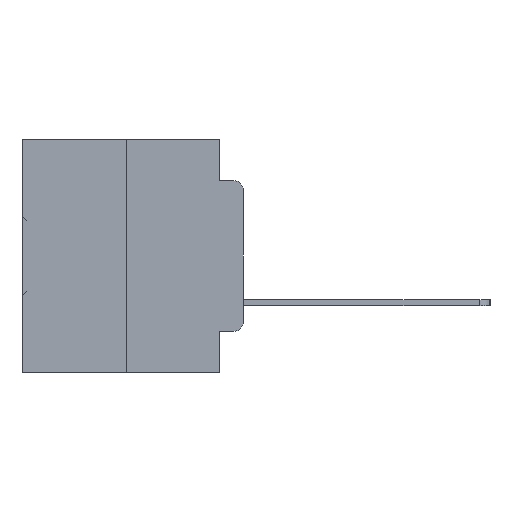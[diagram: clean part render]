
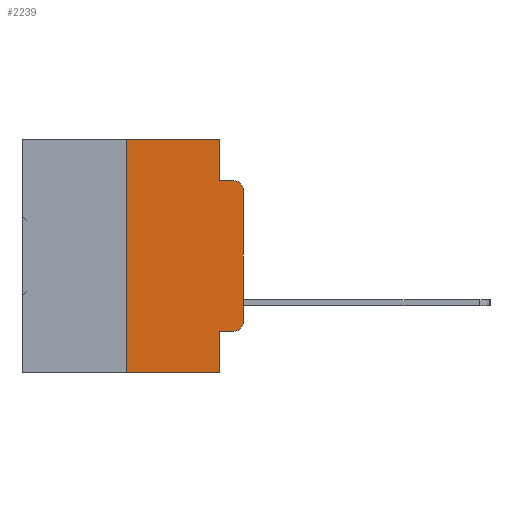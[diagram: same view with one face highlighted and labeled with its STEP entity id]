
A CAD part, left-side view. The second image highlights one B-rep face of the part: STEP entity #2239.
In plain terms, the highlighted planar face has unit normal (-1, 0, 0).
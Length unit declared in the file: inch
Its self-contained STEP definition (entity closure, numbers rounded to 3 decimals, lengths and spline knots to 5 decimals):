
#997 = CARTESIAN_POINT ( 'NONE',  ( 0., 0.051, 0. ) ) ;
#1049 = VECTOR ( 'NONE', #16141, 39.37008 ) ;
#1547 = CIRCLE ( 'NONE', #30281, 0.02 ) ;
#1980 = EDGE_CURVE ( 'NONE', #6962, #26401, #17371, .T. ) ;
#2239 = ADVANCED_FACE ( 'NONE', ( #8444 ), #26455, .F. ) ;
#2429 = CARTESIAN_POINT ( 'NONE',  ( 0., 0.02, -0.1085 ) ) ;
#3225 = DIRECTION ( 'NONE',  ( -1., 0., 0. ) ) ;
#4237 = ORIENTED_EDGE ( 'NONE', *, *, #25578, .T. ) ;
#5030 = VERTEX_POINT ( 'NONE', #24433 ) ;
#5188 = VERTEX_POINT ( 'NONE', #13718 ) ;
#5341 = DIRECTION ( 'NONE',  ( 0., 0., -1. ) ) ;
#5739 = LINE ( 'NONE', #11462, #27465 ) ;
#6173 = LINE ( 'NONE', #27408, #26995 ) ;
#6200 = CARTESIAN_POINT ( 'NONE',  ( 0., 0.25, -0.5 ) ) ;
#6962 = VERTEX_POINT ( 'NONE', #7431 ) ;
#7214 = AXIS2_PLACEMENT_3D ( 'NONE', #20327, #3225, #23152 ) ;
#7288 = EDGE_CURVE ( 'NONE', #20079, #12696, #6173, .T. ) ;
#7431 = CARTESIAN_POINT ( 'NONE',  ( 0., 0.051, -0.4115 ) ) ;
#8252 = ORIENTED_EDGE ( 'NONE', *, *, #18766, .F. ) ;
#8444 = FACE_OUTER_BOUND ( 'NONE', #18345, .T. ) ;
#9199 = VERTEX_POINT ( 'NONE', #16637 ) ;
#9773 = EDGE_CURVE ( 'NONE', #5188, #16081, #17669, .T. ) ;
#9818 = VECTOR ( 'NONE', #31308, 39.37008 ) ;
#11427 = ORIENTED_EDGE ( 'NONE', *, *, #23356, .T. ) ;
#11462 = CARTESIAN_POINT ( 'NONE',  ( 0., 0., 0. ) ) ;
#12016 = LINE ( 'NONE', #997, #26105 ) ;
#12602 = CARTESIAN_POINT ( 'NONE',  ( 0., 0., -0.1085 ) ) ;
#12696 = VERTEX_POINT ( 'NONE', #33293 ) ;
#13718 = CARTESIAN_POINT ( 'NONE',  ( 0., 0.25, 0. ) ) ;
#14218 = LINE ( 'NONE', #17754, #20815 ) ;
#14300 = CIRCLE ( 'NONE', #7214, 0.02 ) ;
#16081 = VERTEX_POINT ( 'NONE', #24579 ) ;
#16141 = DIRECTION ( 'NONE',  ( 0., -1., 0. ) ) ;
#16235 = DIRECTION ( 'NONE',  ( 0., -1., 0. ) ) ;
#16310 = ORIENTED_EDGE ( 'NONE', *, *, #16898, .F. ) ;
#16349 = ORIENTED_EDGE ( 'NONE', *, *, #26290, .F. ) ;
#16637 = CARTESIAN_POINT ( 'NONE',  ( 0., 0.051, -0.5 ) ) ;
#16790 = VECTOR ( 'NONE', #16235, 39.37008 ) ;
#16898 = EDGE_CURVE ( 'NONE', #16081, #20079, #33378, .T. ) ;
#17371 = LINE ( 'NONE', #33043, #9818 ) ;
#17664 = CARTESIAN_POINT ( 'NONE',  ( 0., 0.051, 0. ) ) ;
#17669 = LINE ( 'NONE', #24572, #16790 ) ;
#17754 = CARTESIAN_POINT ( 'NONE',  ( 0., 0.25, 0. ) ) ;
#18345 = EDGE_LOOP ( 'NONE', ( #11427, #32995, #31238, #16310, #24193, #8252, #22427, #16349, #35174, #4237 ) ) ;
#18766 = EDGE_CURVE ( 'NONE', #35471, #5188, #14218, .T. ) ;
#19142 = EDGE_CURVE ( 'NONE', #32050, #12696, #1547, .T. ) ;
#19979 = DIRECTION ( 'NONE',  ( 0., 0., 1. ) ) ;
#20079 = VERTEX_POINT ( 'NONE', #20961 ) ;
#20327 = CARTESIAN_POINT ( 'NONE',  ( 0., 0.02, -0.3915 ) ) ;
#20815 = VECTOR ( 'NONE', #34530, 39.37008 ) ;
#20961 = CARTESIAN_POINT ( 'NONE',  ( 0., 0.051, -0.0885 ) ) ;
#22370 = DIRECTION ( 'NONE',  ( -1., 0., 0. ) ) ;
#22427 = ORIENTED_EDGE ( 'NONE', *, *, #28146, .T. ) ;
#23152 = DIRECTION ( 'NONE',  ( 0., 0., -1. ) ) ;
#23298 = DIRECTION ( 'NONE',  ( 0., 0., -1. ) ) ;
#23356 = EDGE_CURVE ( 'NONE', #5030, #32050, #5739, .T. ) ;
#23667 = AXIS2_PLACEMENT_3D ( 'NONE', #31352, #30116, #32804 ) ;
#23840 = DIRECTION ( 'NONE',  ( 0., 0., -1. ) ) ;
#24193 = ORIENTED_EDGE ( 'NONE', *, *, #9773, .F. ) ;
#24433 = CARTESIAN_POINT ( 'NONE',  ( 0., 0., -0.3915 ) ) ;
#24572 = CARTESIAN_POINT ( 'NONE',  ( 0., 0.473, 0. ) ) ;
#24579 = CARTESIAN_POINT ( 'NONE',  ( 0., 0.051, 0. ) ) ;
#25578 = EDGE_CURVE ( 'NONE', #26401, #5030, #14300, .T. ) ;
#26105 = VECTOR ( 'NONE', #23840, 39.37008 ) ;
#26290 = EDGE_CURVE ( 'NONE', #6962, #9199, #12016, .T. ) ;
#26401 = VERTEX_POINT ( 'NONE', #27132 ) ;
#26455 = PLANE ( 'NONE',  #23667 ) ;
#26995 = VECTOR ( 'NONE', #27290, 39.37008 ) ;
#27132 = CARTESIAN_POINT ( 'NONE',  ( 0., 0.02, -0.4115 ) ) ;
#27290 = DIRECTION ( 'NONE',  ( 0., -1., 0. ) ) ;
#27408 = CARTESIAN_POINT ( 'NONE',  ( 0., 0.051, -0.0885 ) ) ;
#27465 = VECTOR ( 'NONE', #19979, 39.37008 ) ;
#28146 = EDGE_CURVE ( 'NONE', #35471, #9199, #35197, .T. ) ;
#30116 = DIRECTION ( 'NONE',  ( 1., 0., 0. ) ) ;
#30281 = AXIS2_PLACEMENT_3D ( 'NONE', #2429, #22370, #5341 ) ;
#31238 = ORIENTED_EDGE ( 'NONE', *, *, #7288, .F. ) ;
#31308 = DIRECTION ( 'NONE',  ( 0., -1., 0. ) ) ;
#31352 = CARTESIAN_POINT ( 'NONE',  ( 0., 0.473, 0. ) ) ;
#32050 = VERTEX_POINT ( 'NONE', #12602 ) ;
#32510 = VECTOR ( 'NONE', #23298, 39.37008 ) ;
#32804 = DIRECTION ( 'NONE',  ( 0., 0., -1. ) ) ;
#32939 = CARTESIAN_POINT ( 'NONE',  ( 0., 0.473, -0.5 ) ) ;
#32995 = ORIENTED_EDGE ( 'NONE', *, *, #19142, .T. ) ;
#33043 = CARTESIAN_POINT ( 'NONE',  ( 0., 0.051, -0.4115 ) ) ;
#33293 = CARTESIAN_POINT ( 'NONE',  ( 0., 0.02, -0.0885 ) ) ;
#33378 = LINE ( 'NONE', #17664, #32510 ) ;
#34530 = DIRECTION ( 'NONE',  ( 0., 0., 1. ) ) ;
#35174 = ORIENTED_EDGE ( 'NONE', *, *, #1980, .T. ) ;
#35197 = LINE ( 'NONE', #32939, #1049 ) ;
#35471 = VERTEX_POINT ( 'NONE', #6200 ) ;
